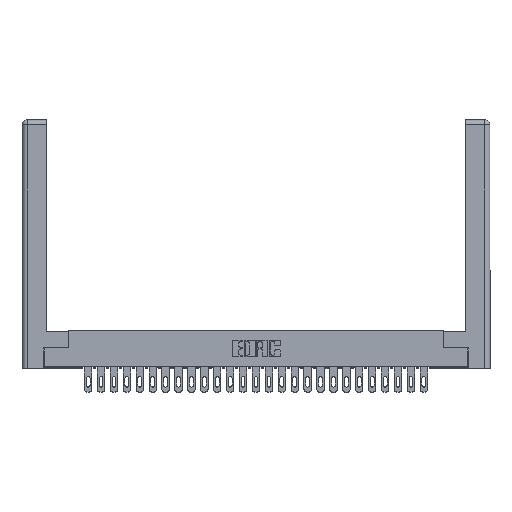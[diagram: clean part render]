
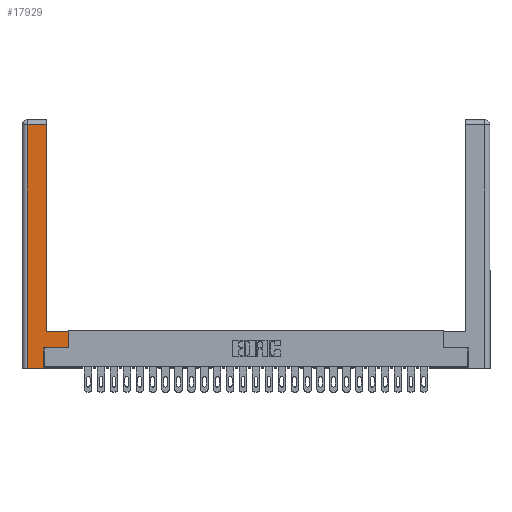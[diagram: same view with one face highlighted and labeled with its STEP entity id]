
A CAD part, top view. The second image highlights one B-rep face of the part: STEP entity #17929.
In plain terms, the highlighted planar face has unit normal (0, 0, 1).
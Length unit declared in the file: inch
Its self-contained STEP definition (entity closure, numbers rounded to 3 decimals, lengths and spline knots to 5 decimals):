
#345 = VECTOR ( 'NONE', #14478, 39.37008 ) ;
#1343 = CARTESIAN_POINT ( 'NONE',  ( 0.295, 0.45, 0. ) ) ;
#2238 = VERTEX_POINT ( 'NONE', #9152 ) ;
#2528 = VERTEX_POINT ( 'NONE', #19290 ) ;
#3550 = CARTESIAN_POINT ( 'NONE',  ( 0.265, 0.245, 0. ) ) ;
#3896 = ORIENTED_EDGE ( 'NONE', *, *, #17605, .T. ) ;
#4113 = EDGE_LOOP ( 'NONE', ( #26868, #8227, #3896, #24879, #8811, #11626, #9083, #9287 ) ) ;
#4329 = EDGE_CURVE ( 'NONE', #27033, #14074, #30263, .T. ) ;
#4437 = CARTESIAN_POINT ( 'NONE',  ( 0.295, 2.94, 0. ) ) ;
#4909 = LINE ( 'NONE', #26874, #14314 ) ;
#5435 = AXIS2_PLACEMENT_3D ( 'NONE', #13893, #27140, #32118 ) ;
#6301 = DIRECTION ( 'NONE',  ( -1., 0., 0. ) ) ;
#7375 = EDGE_CURVE ( 'NONE', #31392, #2528, #24506, .T. ) ;
#8227 = ORIENTED_EDGE ( 'NONE', *, *, #7375, .T. ) ;
#8811 = ORIENTED_EDGE ( 'NONE', *, *, #4329, .T. ) ;
#9003 = DIRECTION ( 'NONE',  ( 0., 1., 0. ) ) ;
#9004 = FACE_OUTER_BOUND ( 'NONE', #4113, .T. ) ;
#9083 = ORIENTED_EDGE ( 'NONE', *, *, #12849, .T. ) ;
#9091 = EDGE_CURVE ( 'NONE', #27442, #30192, #4909, .T. ) ;
#9152 = CARTESIAN_POINT ( 'NONE',  ( 0.0615, 0., 0. ) ) ;
#9287 = ORIENTED_EDGE ( 'NONE', *, *, #9091, .T. ) ;
#10663 = LINE ( 'NONE', #19477, #16737 ) ;
#10894 = LINE ( 'NONE', #14771, #24670 ) ;
#10927 = VERTEX_POINT ( 'NONE', #19569 ) ;
#11626 = ORIENTED_EDGE ( 'NONE', *, *, #24246, .T. ) ;
#11919 = VECTOR ( 'NONE', #6301, 39.37008 ) ;
#12849 = EDGE_CURVE ( 'NONE', #10927, #27442, #10663, .T. ) ;
#13724 = DIRECTION ( 'NONE',  ( 0., 1., 0. ) ) ;
#13893 = CARTESIAN_POINT ( 'NONE',  ( 0., 0., 0. ) ) ;
#14001 = PLANE ( 'NONE',  #5435 ) ;
#14074 = VERTEX_POINT ( 'NONE', #3550 ) ;
#14314 = VECTOR ( 'NONE', #26173, 39.37008 ) ;
#14440 = CARTESIAN_POINT ( 'NONE',  ( 0.0615, 0., 0. ) ) ;
#14478 = DIRECTION ( 'NONE',  ( 0., 1., 0. ) ) ;
#14771 = CARTESIAN_POINT ( 'NONE',  ( 0.565, 0.245, 0. ) ) ;
#15551 = VECTOR ( 'NONE', #16916, 39.37008 ) ;
#16276 = LINE ( 'NONE', #27060, #345 ) ;
#16737 = VECTOR ( 'NONE', #9003, 39.37008 ) ;
#16916 = DIRECTION ( 'NONE',  ( 0., -1., 0. ) ) ;
#17605 = EDGE_CURVE ( 'NONE', #2528, #2238, #28315, .T. ) ;
#17929 = ADVANCED_FACE ( 'NONE', ( #9004 ), #14001, .F. ) ;
#18365 = EDGE_CURVE ( 'NONE', #30192, #31392, #16276, .T. ) ;
#19290 = CARTESIAN_POINT ( 'NONE',  ( 0.0615, 2.94, 0. ) ) ;
#19477 = CARTESIAN_POINT ( 'NONE',  ( 0.565, 0.45, 0. ) ) ;
#19569 = CARTESIAN_POINT ( 'NONE',  ( 0.565, 0.245, 0. ) ) ;
#20545 = LINE ( 'NONE', #21240, #21748 ) ;
#21240 = CARTESIAN_POINT ( 'NONE',  ( 0.265, 0., 0. ) ) ;
#21347 = DIRECTION ( 'NONE',  ( 1., 0., 0. ) ) ;
#21748 = VECTOR ( 'NONE', #21347, 39.37008 ) ;
#21984 = CARTESIAN_POINT ( 'NONE',  ( 0.265, 0., 0. ) ) ;
#22132 = DIRECTION ( 'NONE',  ( 1., 0., 0. ) ) ;
#23929 = CARTESIAN_POINT ( 'NONE',  ( 0.265, 0.245, 0. ) ) ;
#24246 = EDGE_CURVE ( 'NONE', #14074, #10927, #10894, .T. ) ;
#24506 = LINE ( 'NONE', #32168, #11919 ) ;
#24670 = VECTOR ( 'NONE', #22132, 39.37008 ) ;
#24879 = ORIENTED_EDGE ( 'NONE', *, *, #31542, .T. ) ;
#26173 = DIRECTION ( 'NONE',  ( -1., 0., 0. ) ) ;
#26370 = CARTESIAN_POINT ( 'NONE',  ( 0.565, 0.45, 0. ) ) ;
#26868 = ORIENTED_EDGE ( 'NONE', *, *, #18365, .T. ) ;
#26874 = CARTESIAN_POINT ( 'NONE',  ( 0.295, 0.45, 0. ) ) ;
#27033 = VERTEX_POINT ( 'NONE', #21984 ) ;
#27060 = CARTESIAN_POINT ( 'NONE',  ( 0.295, 3., 0. ) ) ;
#27140 = DIRECTION ( 'NONE',  ( 0., 0., -1. ) ) ;
#27442 = VERTEX_POINT ( 'NONE', #26370 ) ;
#28315 = LINE ( 'NONE', #14440, #15551 ) ;
#30192 = VERTEX_POINT ( 'NONE', #1343 ) ;
#30263 = LINE ( 'NONE', #23929, #30665 ) ;
#30665 = VECTOR ( 'NONE', #13724, 39.37008 ) ;
#31392 = VERTEX_POINT ( 'NONE', #4437 ) ;
#31542 = EDGE_CURVE ( 'NONE', #2238, #27033, #20545, .T. ) ;
#32118 = DIRECTION ( 'NONE',  ( -1., 0., 0. ) ) ;
#32168 = CARTESIAN_POINT ( 'NONE',  ( 0.0615, 2.94, 0. ) ) ;
